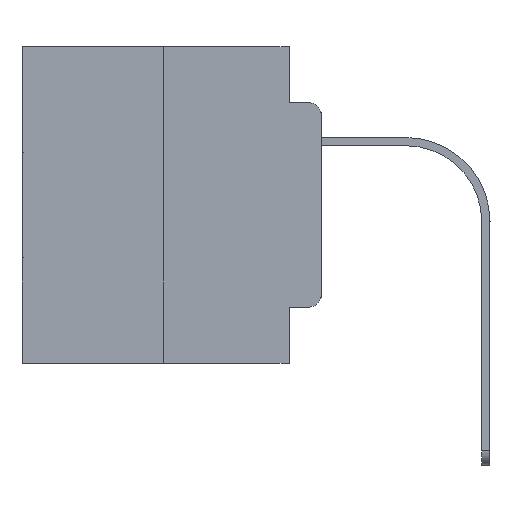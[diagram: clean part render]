
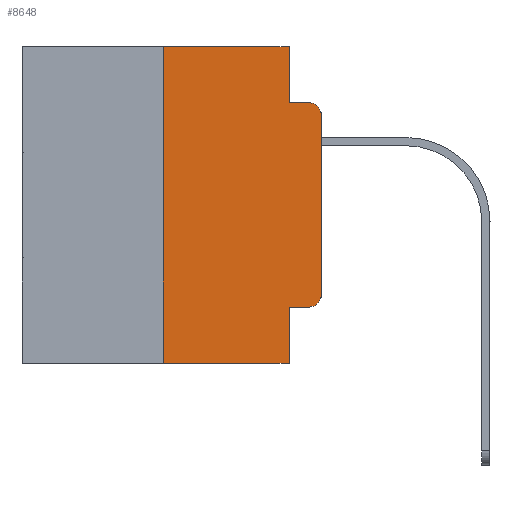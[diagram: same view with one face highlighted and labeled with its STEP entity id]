
A CAD part, left-side view. The second image highlights one B-rep face of the part: STEP entity #8648.
In plain terms, the highlighted planar face has unit normal (-1, 0, 0).
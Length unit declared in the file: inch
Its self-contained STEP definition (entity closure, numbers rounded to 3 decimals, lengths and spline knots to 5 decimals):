
#39 = LINE ( 'NONE', #19287, #24501 ) ;
#80 = AXIS2_PLACEMENT_3D ( 'NONE', #10474, #8279, #25055 ) ;
#418 = VERTEX_POINT ( 'NONE', #7100 ) ;
#487 = VERTEX_POINT ( 'NONE', #2438 ) ;
#632 = VERTEX_POINT ( 'NONE', #2147 ) ;
#938 = ORIENTED_EDGE ( 'NONE', *, *, #24112, .F. ) ;
#1249 = EDGE_CURVE ( 'NONE', #14795, #24373, #1722, .T. ) ;
#1460 = ORIENTED_EDGE ( 'NONE', *, *, #19941, .F. ) ;
#1599 = DIRECTION ( 'NONE',  ( -1., 0., 0. ) ) ;
#1611 = DIRECTION ( 'NONE',  ( 0., 0., -1. ) ) ;
#1704 = EDGE_CURVE ( 'NONE', #14795, #26604, #39, .T. ) ;
#1722 = LINE ( 'NONE', #8027, #21564 ) ;
#1792 = CARTESIAN_POINT ( 'NONE',  ( 0., 0.02, -0.1085 ) ) ;
#2026 = EDGE_CURVE ( 'NONE', #9903, #11199, #4858, .T. ) ;
#2033 = EDGE_LOOP ( 'NONE', ( #4802, #3956, #1460, #20214, #15386, #10094, #24377, #938, #14614, #19207 ) ) ;
#2147 = CARTESIAN_POINT ( 'NONE',  ( 0., 0.02, -0.4115 ) ) ;
#2438 = CARTESIAN_POINT ( 'NONE',  ( 0., 0.051, -0.0885 ) ) ;
#2624 = LINE ( 'NONE', #17385, #21906 ) ;
#2816 = VECTOR ( 'NONE', #12011, 39.37008 ) ;
#2956 = CARTESIAN_POINT ( 'NONE',  ( 0., 0.25, -0.5 ) ) ;
#3743 = VECTOR ( 'NONE', #13164, 39.37008 ) ;
#3956 = ORIENTED_EDGE ( 'NONE', *, *, #2026, .T. ) ;
#4542 = EDGE_CURVE ( 'NONE', #24373, #418, #8554, .T. ) ;
#4802 = ORIENTED_EDGE ( 'NONE', *, *, #10360, .T. ) ;
#4858 = CIRCLE ( 'NONE', #13633, 0.02 ) ;
#5426 = CARTESIAN_POINT ( 'NONE',  ( 0., 0.02, -0.3915 ) ) ;
#5681 = VECTOR ( 'NONE', #24174, 39.37008 ) ;
#6323 = DIRECTION ( 'NONE',  ( 0., -1., 0. ) ) ;
#6506 = CARTESIAN_POINT ( 'NONE',  ( 0., 0.02, -0.0885 ) ) ;
#7100 = CARTESIAN_POINT ( 'NONE',  ( 0., 0.051, 0. ) ) ;
#7535 = CARTESIAN_POINT ( 'NONE',  ( 0., 0.051, 0. ) ) ;
#7912 = LINE ( 'NONE', #8446, #13038 ) ;
#8027 = CARTESIAN_POINT ( 'NONE',  ( 0., 0.25, 0. ) ) ;
#8279 = DIRECTION ( 'NONE',  ( 1., 0., 0. ) ) ;
#8446 = CARTESIAN_POINT ( 'NONE',  ( 0., 0.051, 0. ) ) ;
#8545 = FACE_OUTER_BOUND ( 'NONE', #2033, .T. ) ;
#8554 = LINE ( 'NONE', #16889, #14900 ) ;
#8648 = ADVANCED_FACE ( 'NONE', ( #8545 ), #22889, .F. ) ;
#9903 = VERTEX_POINT ( 'NONE', #26971 ) ;
#10094 = ORIENTED_EDGE ( 'NONE', *, *, #1249, .F. ) ;
#10360 = EDGE_CURVE ( 'NONE', #25608, #9903, #23105, .T. ) ;
#10474 = CARTESIAN_POINT ( 'NONE',  ( 0., 0.473, 0. ) ) ;
#10617 = DIRECTION ( 'NONE',  ( 0., 0., 1. ) ) ;
#11199 = VERTEX_POINT ( 'NONE', #6506 ) ;
#11232 = VERTEX_POINT ( 'NONE', #18823 ) ;
#11611 = DIRECTION ( 'NONE',  ( 0., 0., -1. ) ) ;
#12011 = DIRECTION ( 'NONE',  ( 0., -1., 0. ) ) ;
#13038 = VECTOR ( 'NONE', #1611, 39.37008 ) ;
#13067 = DIRECTION ( 'NONE',  ( 0., -1., 0. ) ) ;
#13164 = DIRECTION ( 'NONE',  ( 0., 0., 1. ) ) ;
#13553 = EDGE_CURVE ( 'NONE', #632, #25608, #22810, .T. ) ;
#13633 = AXIS2_PLACEMENT_3D ( 'NONE', #1792, #22690, #22291 ) ;
#14370 = EDGE_CURVE ( 'NONE', #418, #487, #26196, .T. ) ;
#14614 = ORIENTED_EDGE ( 'NONE', *, *, #16683, .T. ) ;
#14795 = VERTEX_POINT ( 'NONE', #2956 ) ;
#14900 = VECTOR ( 'NONE', #13067, 39.37008 ) ;
#15386 = ORIENTED_EDGE ( 'NONE', *, *, #4542, .F. ) ;
#15831 = CARTESIAN_POINT ( 'NONE',  ( 0., 0.051, -0.0885 ) ) ;
#15963 = LINE ( 'NONE', #15831, #2816 ) ;
#16683 = EDGE_CURVE ( 'NONE', #11232, #632, #2624, .T. ) ;
#16724 = AXIS2_PLACEMENT_3D ( 'NONE', #5426, #1599, #11611 ) ;
#16889 = CARTESIAN_POINT ( 'NONE',  ( 0., 0.473, 0. ) ) ;
#17385 = CARTESIAN_POINT ( 'NONE',  ( 0., 0.051, -0.4115 ) ) ;
#18823 = CARTESIAN_POINT ( 'NONE',  ( 0., 0.051, -0.4115 ) ) ;
#19207 = ORIENTED_EDGE ( 'NONE', *, *, #13553, .T. ) ;
#19287 = CARTESIAN_POINT ( 'NONE',  ( 0., 0.473, -0.5 ) ) ;
#19941 = EDGE_CURVE ( 'NONE', #487, #11199, #15963, .T. ) ;
#20214 = ORIENTED_EDGE ( 'NONE', *, *, #14370, .F. ) ;
#21564 = VECTOR ( 'NONE', #10617, 39.37008 ) ;
#21807 = CARTESIAN_POINT ( 'NONE',  ( 0., 0.25, 0. ) ) ;
#21906 = VECTOR ( 'NONE', #25291, 39.37008 ) ;
#22291 = DIRECTION ( 'NONE',  ( 0., 0., -1. ) ) ;
#22682 = CARTESIAN_POINT ( 'NONE',  ( 0., 0.051, -0.5 ) ) ;
#22690 = DIRECTION ( 'NONE',  ( -1., 0., 0. ) ) ;
#22810 = CIRCLE ( 'NONE', #16724, 0.02 ) ;
#22889 = PLANE ( 'NONE',  #80 ) ;
#23105 = LINE ( 'NONE', #23504, #3743 ) ;
#23504 = CARTESIAN_POINT ( 'NONE',  ( 0., 0., 0. ) ) ;
#23602 = CARTESIAN_POINT ( 'NONE',  ( 0., 0., -0.3915 ) ) ;
#24112 = EDGE_CURVE ( 'NONE', #11232, #26604, #7912, .T. ) ;
#24174 = DIRECTION ( 'NONE',  ( 0., 0., -1. ) ) ;
#24373 = VERTEX_POINT ( 'NONE', #21807 ) ;
#24377 = ORIENTED_EDGE ( 'NONE', *, *, #1704, .T. ) ;
#24501 = VECTOR ( 'NONE', #6323, 39.37008 ) ;
#25055 = DIRECTION ( 'NONE',  ( 0., 0., -1. ) ) ;
#25291 = DIRECTION ( 'NONE',  ( 0., -1., 0. ) ) ;
#25608 = VERTEX_POINT ( 'NONE', #23602 ) ;
#26196 = LINE ( 'NONE', #7535, #5681 ) ;
#26604 = VERTEX_POINT ( 'NONE', #22682 ) ;
#26971 = CARTESIAN_POINT ( 'NONE',  ( 0., 0., -0.1085 ) ) ;
